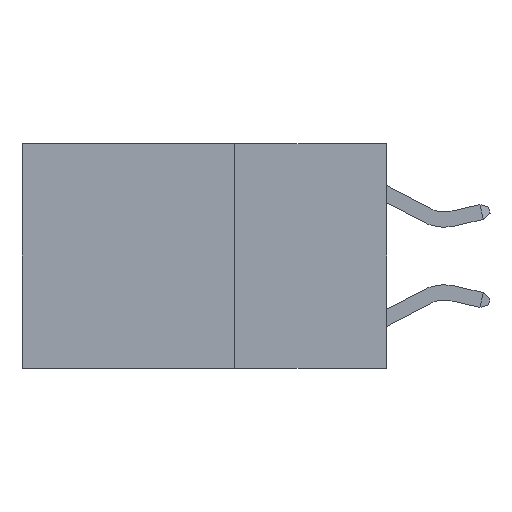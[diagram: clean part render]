
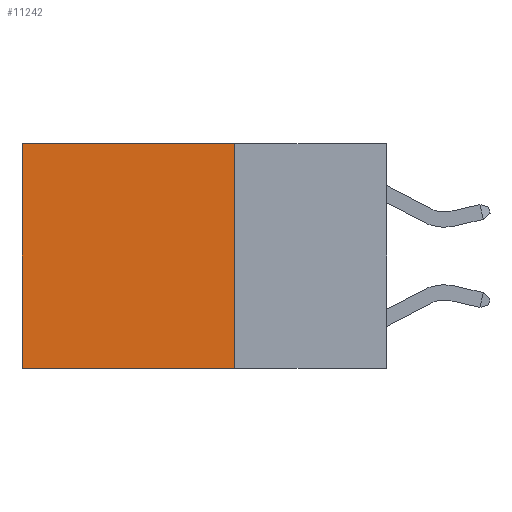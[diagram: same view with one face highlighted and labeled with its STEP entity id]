
A CAD part, left-side view. The second image highlights one B-rep face of the part: STEP entity #11242.
In plain terms, the highlighted planar face has unit normal (-1, 0, 0).
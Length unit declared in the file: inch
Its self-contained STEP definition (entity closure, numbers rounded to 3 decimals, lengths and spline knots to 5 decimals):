
#80 = ORIENTED_EDGE ( 'NONE', *, *, #3856, .T. ) ;
#241 = DIRECTION ( 'NONE',  ( 0., 0., -1. ) ) ;
#519 = CARTESIAN_POINT ( 'NONE',  ( 0.2625, 0.25, 0. ) ) ;
#1122 = ORIENTED_EDGE ( 'NONE', *, *, #5498, .F. ) ;
#3071 = LINE ( 'NONE', #519, #13726 ) ;
#3239 = DIRECTION ( 'NONE',  ( 0., 0., -1. ) ) ;
#3779 = LINE ( 'NONE', #16828, #14852 ) ;
#3809 = PLANE ( 'NONE',  #8272 ) ;
#3856 = EDGE_CURVE ( 'NONE', #11086, #13808, #3779, .T. ) ;
#5443 = EDGE_CURVE ( 'NONE', #11086, #12435, #3071, .T. ) ;
#5498 = EDGE_CURVE ( 'NONE', #12435, #15107, #10031, .T. ) ;
#6314 = VECTOR ( 'NONE', #16027, 39.37008 ) ;
#7215 = ORIENTED_EDGE ( 'NONE', *, *, #10978, .T. ) ;
#7325 = CARTESIAN_POINT ( 'NONE',  ( 0.2625, 0.6, 0. ) ) ;
#7685 = CARTESIAN_POINT ( 'NONE',  ( 0.2625, 0.25, 0. ) ) ;
#8272 = AXIS2_PLACEMENT_3D ( 'NONE', #9246, #13417, #9299 ) ;
#9246 = CARTESIAN_POINT ( 'NONE',  ( 0.2625, 0.25, 0. ) ) ;
#9299 = DIRECTION ( 'NONE',  ( 0., 0., -1. ) ) ;
#9418 = ORIENTED_EDGE ( 'NONE', *, *, #5443, .F. ) ;
#9816 = DIRECTION ( 'NONE',  ( 0., 1., 0. ) ) ;
#9935 = EDGE_LOOP ( 'NONE', ( #7215, #1122, #9418, #80 ) ) ;
#10031 = LINE ( 'NONE', #13328, #6314 ) ;
#10960 = LINE ( 'NONE', #7325, #15698 ) ;
#10978 = EDGE_CURVE ( 'NONE', #13808, #15107, #10960, .T. ) ;
#11086 = VERTEX_POINT ( 'NONE', #7685 ) ;
#11242 = ADVANCED_FACE ( 'NONE', ( #13762 ), #3809, .F. ) ;
#12435 = VERTEX_POINT ( 'NONE', #14615 ) ;
#13328 = CARTESIAN_POINT ( 'NONE',  ( 0.2625, 0.25, -0.37 ) ) ;
#13417 = DIRECTION ( 'NONE',  ( 1., 0., 0. ) ) ;
#13726 = VECTOR ( 'NONE', #3239, 39.37008 ) ;
#13762 = FACE_OUTER_BOUND ( 'NONE', #9935, .T. ) ;
#13808 = VERTEX_POINT ( 'NONE', #17277 ) ;
#14615 = CARTESIAN_POINT ( 'NONE',  ( 0.2625, 0.25, -0.37 ) ) ;
#14852 = VECTOR ( 'NONE', #9816, 39.37008 ) ;
#15107 = VERTEX_POINT ( 'NONE', #16110 ) ;
#15698 = VECTOR ( 'NONE', #241, 39.37008 ) ;
#16027 = DIRECTION ( 'NONE',  ( 0., 1., 0. ) ) ;
#16110 = CARTESIAN_POINT ( 'NONE',  ( 0.2625, 0.6, -0.37 ) ) ;
#16828 = CARTESIAN_POINT ( 'NONE',  ( 0.2625, 0.25, 0. ) ) ;
#17277 = CARTESIAN_POINT ( 'NONE',  ( 0.2625, 0.6, 0. ) ) ;
